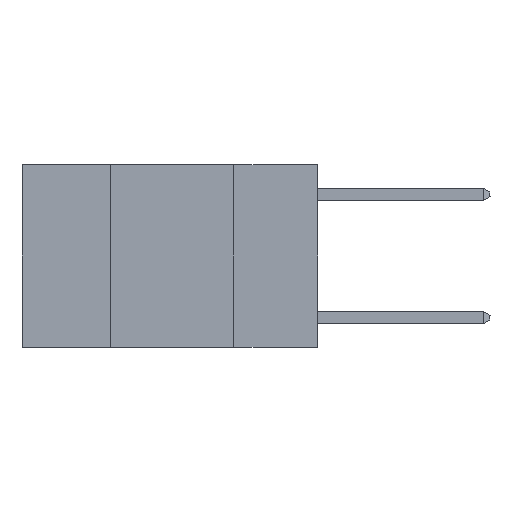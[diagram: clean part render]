
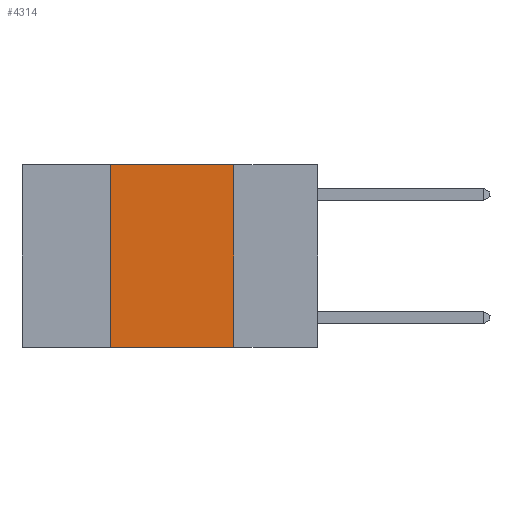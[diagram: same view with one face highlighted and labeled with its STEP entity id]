
A CAD part, left-side view. The second image highlights one B-rep face of the part: STEP entity #4314.
In plain terms, the highlighted planar face has unit normal (-1, 0, 0).
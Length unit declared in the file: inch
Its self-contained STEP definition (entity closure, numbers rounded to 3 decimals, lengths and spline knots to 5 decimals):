
#1722 = DIRECTION ( 'NONE',  ( 0., -1., 0. ) ) ;
#1843 = FACE_OUTER_BOUND ( 'NONE', #26249, .T. ) ;
#2505 = ORIENTED_EDGE ( 'NONE', *, *, #3759, .F. ) ;
#2830 = AXIS2_PLACEMENT_3D ( 'NONE', #7775, #17107, #3123 ) ;
#2886 = DIRECTION ( 'NONE',  ( 0., 0., -1. ) ) ;
#3123 = DIRECTION ( 'NONE',  ( 0., 0., -1. ) ) ;
#3759 = EDGE_CURVE ( 'NONE', #8448, #12032, #4839, .T. ) ;
#3996 = LINE ( 'NONE', #25273, #21900 ) ;
#4011 = ORIENTED_EDGE ( 'NONE', *, *, #20771, .F. ) ;
#4314 = ADVANCED_FACE ( 'NONE', ( #1843 ), #14787, .F. ) ;
#4839 = LINE ( 'NONE', #28676, #16528 ) ;
#7775 = CARTESIAN_POINT ( 'NONE',  ( 0., 0.6, 0. ) ) ;
#8448 = VERTEX_POINT ( 'NONE', #16643 ) ;
#9463 = EDGE_CURVE ( 'NONE', #19564, #9505, #3996, .T. ) ;
#9505 = VERTEX_POINT ( 'NONE', #25370 ) ;
#10609 = ORIENTED_EDGE ( 'NONE', *, *, #12776, .T. ) ;
#11312 = DIRECTION ( 'NONE',  ( 0., 0., 1. ) ) ;
#12032 = VERTEX_POINT ( 'NONE', #20458 ) ;
#12776 = EDGE_CURVE ( 'NONE', #19564, #12032, #25683, .T. ) ;
#13423 = CARTESIAN_POINT ( 'NONE',  ( 0., 0.6, 0. ) ) ;
#14787 = PLANE ( 'NONE',  #2830 ) ;
#14890 = LINE ( 'NONE', #13423, #20383 ) ;
#15351 = ORIENTED_EDGE ( 'NONE', *, *, #9463, .F. ) ;
#16528 = VECTOR ( 'NONE', #2886, 39.37008 ) ;
#16643 = CARTESIAN_POINT ( 'NONE',  ( 0., 0.17, 0. ) ) ;
#16760 = CARTESIAN_POINT ( 'NONE',  ( 0., 0.42, -0.37 ) ) ;
#17107 = DIRECTION ( 'NONE',  ( 1., 0., 0. ) ) ;
#18749 = VECTOR ( 'NONE', #22863, 39.37008 ) ;
#19564 = VERTEX_POINT ( 'NONE', #16760 ) ;
#20383 = VECTOR ( 'NONE', #1722, 39.37008 ) ;
#20458 = CARTESIAN_POINT ( 'NONE',  ( 0., 0.17, -0.37 ) ) ;
#20521 = CARTESIAN_POINT ( 'NONE',  ( 0., 0.6, -0.37 ) ) ;
#20771 = EDGE_CURVE ( 'NONE', #9505, #8448, #14890, .T. ) ;
#21900 = VECTOR ( 'NONE', #11312, 39.37008 ) ;
#22863 = DIRECTION ( 'NONE',  ( 0., -1., 0. ) ) ;
#25273 = CARTESIAN_POINT ( 'NONE',  ( 0., 0.42, 0. ) ) ;
#25370 = CARTESIAN_POINT ( 'NONE',  ( 0., 0.42, 0. ) ) ;
#25683 = LINE ( 'NONE', #20521, #18749 ) ;
#26249 = EDGE_LOOP ( 'NONE', ( #2505, #4011, #15351, #10609 ) ) ;
#28676 = CARTESIAN_POINT ( 'NONE',  ( 0., 0.17, 0. ) ) ;
